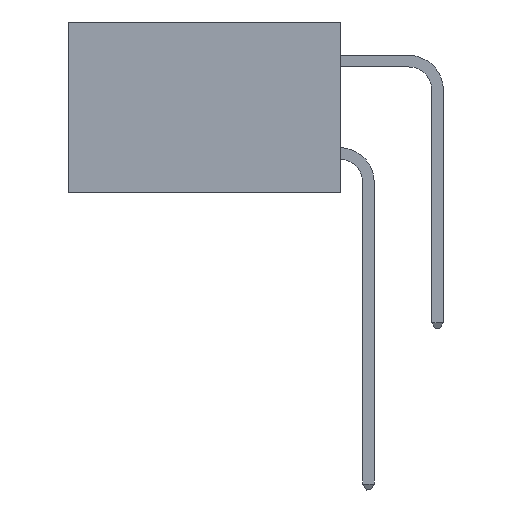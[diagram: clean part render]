
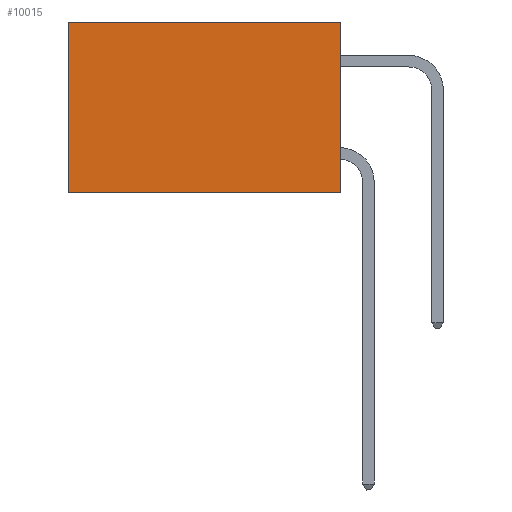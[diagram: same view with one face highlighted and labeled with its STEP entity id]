
A CAD part, left-side view. The second image highlights one B-rep face of the part: STEP entity #10015.
In plain terms, the highlighted planar face has unit normal (-1, 0, 0).
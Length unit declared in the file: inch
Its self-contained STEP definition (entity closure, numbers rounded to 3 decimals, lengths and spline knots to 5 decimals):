
#250 = CARTESIAN_POINT ( 'NONE',  ( 0.277, 0., -0.37 ) ) ;
#706 = VECTOR ( 'NONE', #2707, 39.37008 ) ;
#1461 = VECTOR ( 'NONE', #7373, 39.37008 ) ;
#2707 = DIRECTION ( 'NONE',  ( 0., 1., 0. ) ) ;
#3399 = LINE ( 'NONE', #7217, #24073 ) ;
#3446 = VERTEX_POINT ( 'NONE', #7207 ) ;
#4483 = EDGE_LOOP ( 'NONE', ( #25312, #13338, #8528, #19011 ) ) ;
#5315 = FACE_OUTER_BOUND ( 'NONE', #4483, .T. ) ;
#5683 = CARTESIAN_POINT ( 'NONE',  ( 0.277, 0., 0. ) ) ;
#5799 = LINE ( 'NONE', #10238, #7989 ) ;
#6098 = LINE ( 'NONE', #5683, #706 ) ;
#6104 = EDGE_CURVE ( 'NONE', #3446, #24129, #6098, .T. ) ;
#7207 = CARTESIAN_POINT ( 'NONE',  ( 0.277, 0., 0. ) ) ;
#7217 = CARTESIAN_POINT ( 'NONE',  ( 0.277, 0., -0.37 ) ) ;
#7373 = DIRECTION ( 'NONE',  ( 0., 1., 0. ) ) ;
#7488 = AXIS2_PLACEMENT_3D ( 'NONE', #21944, #9972, #23899 ) ;
#7938 = PLANE ( 'NONE',  #7488 ) ;
#7989 = VECTOR ( 'NONE', #14244, 39.37008 ) ;
#8528 = ORIENTED_EDGE ( 'NONE', *, *, #9646, .F. ) ;
#9646 = EDGE_CURVE ( 'NONE', #3446, #21695, #3399, .T. ) ;
#9972 = DIRECTION ( 'NONE',  ( 1., 0., 0. ) ) ;
#10015 = ADVANCED_FACE ( 'NONE', ( #5315 ), #7938, .F. ) ;
#10238 = CARTESIAN_POINT ( 'NONE',  ( 0.277, 0.59, -0.37 ) ) ;
#13338 = ORIENTED_EDGE ( 'NONE', *, *, #13527, .F. ) ;
#13527 = EDGE_CURVE ( 'NONE', #21695, #18080, #16865, .T. ) ;
#14244 = DIRECTION ( 'NONE',  ( 0., 0., -1. ) ) ;
#16865 = LINE ( 'NONE', #25287, #1461 ) ;
#18080 = VERTEX_POINT ( 'NONE', #21554 ) ;
#18228 = DIRECTION ( 'NONE',  ( 0., 0., -1. ) ) ;
#18970 = EDGE_CURVE ( 'NONE', #24129, #18080, #5799, .T. ) ;
#19011 = ORIENTED_EDGE ( 'NONE', *, *, #6104, .T. ) ;
#21554 = CARTESIAN_POINT ( 'NONE',  ( 0.277, 0.59, -0.37 ) ) ;
#21695 = VERTEX_POINT ( 'NONE', #250 ) ;
#21944 = CARTESIAN_POINT ( 'NONE',  ( 0.277, 0., -0.37 ) ) ;
#22863 = CARTESIAN_POINT ( 'NONE',  ( 0.277, 0.59, 0. ) ) ;
#23899 = DIRECTION ( 'NONE',  ( 0., 0., -1. ) ) ;
#24073 = VECTOR ( 'NONE', #18228, 39.37008 ) ;
#24129 = VERTEX_POINT ( 'NONE', #22863 ) ;
#25287 = CARTESIAN_POINT ( 'NONE',  ( 0.277, 0., -0.37 ) ) ;
#25312 = ORIENTED_EDGE ( 'NONE', *, *, #18970, .T. ) ;
